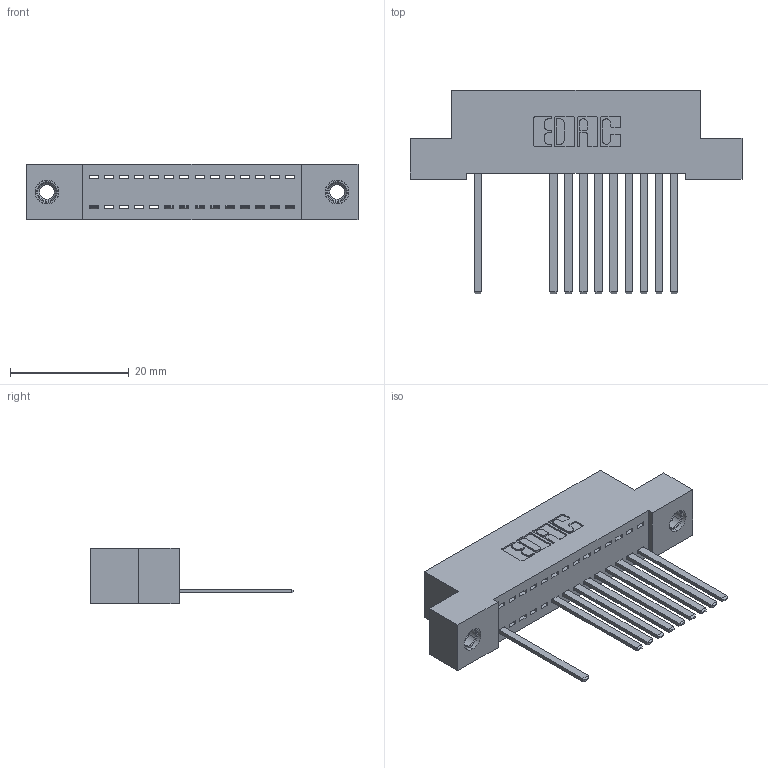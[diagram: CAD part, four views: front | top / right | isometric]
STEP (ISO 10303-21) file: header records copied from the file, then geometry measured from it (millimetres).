
FILE_DESCRIPTION (( 'STEP AP203' ), '1' );
FILE_NAME ('392-014-544-107.STEP', '2018-08-15T00:11:47', ( '' ), ( '' ), 'SwSTEP 2.0', 'SolidWorks 2016', '' );
FILE_SCHEMA (( 'CONFIG_CONTROL_DESIGN' ));
Length unit declared in the file: inch
Products named in the file (4): 345-250-001_345-250-005-103; 392-014-544-107; 342 Part_TI; 345-292-001_345-293-144
Assembly tree (13 placements, depth 2):
  392-014-544-107
    342 Part_TI
    345-292-001_345-293-144  x10
    345-250-001_345-250-005-103  x2
Bounding box: 55.88 x 34.3 x 9.4 mm (x, y, z)
Volume: 4853.8 mm3; surface area: 6729.6 mm2
Topology: 13 solids, 13 shells, 738 faces, 2183 edges, 1434 vertices
Faces by surface type: plane 526, cylinder 196, cone 12, torus 4
Entity records: 12922 total; most frequent: CARTESIAN_POINT 2231, ORIENTED_EDGE 2178, DIRECTION 1963, EDGE_CURVE 1089, VECTOR 945, LINE 945, VERTEX_POINT 720, AXIS2_PLACEMENT_3D 509
